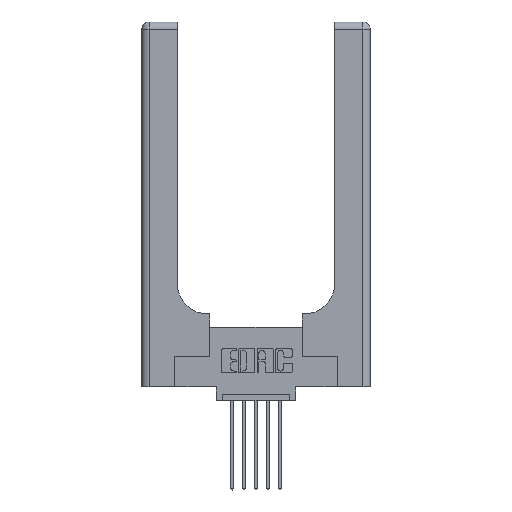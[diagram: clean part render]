
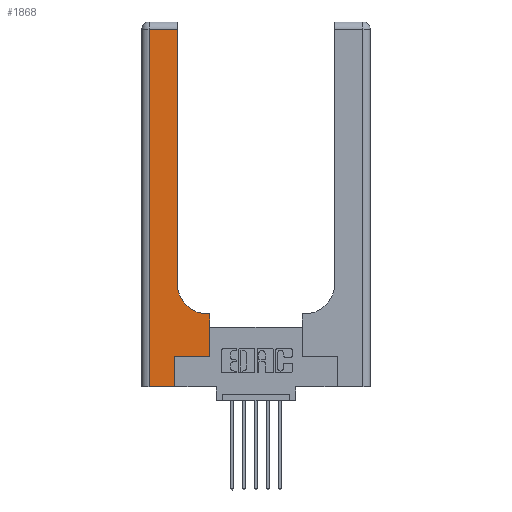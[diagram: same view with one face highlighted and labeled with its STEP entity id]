
A CAD part, top view. The second image highlights one B-rep face of the part: STEP entity #1868.
In plain terms, the highlighted planar face has unit normal (0, 0, 1).
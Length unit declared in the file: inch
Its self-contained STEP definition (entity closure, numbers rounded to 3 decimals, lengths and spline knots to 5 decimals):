
#275 = VERTEX_POINT ( 'NONE', #4577 ) ;
#542 = VECTOR ( 'NONE', #3046, 39.37008 ) ;
#587 = VERTEX_POINT ( 'NONE', #5018 ) ;
#690 = CARTESIAN_POINT ( 'NONE',  ( 0.269, 0.25, 0.37 ) ) ;
#755 = CARTESIAN_POINT ( 'NONE',  ( 0.2915, 0.6, 0.37 ) ) ;
#831 = CARTESIAN_POINT ( 'NONE',  ( 0.269, 0., 0.37 ) ) ;
#941 = CARTESIAN_POINT ( 'NONE',  ( 0.2915, 3., 0.37 ) ) ;
#1002 = DIRECTION ( 'NONE',  ( 0., 0., -1. ) ) ;
#1436 = DIRECTION ( 'NONE',  ( -1., 0., 0. ) ) ;
#1779 = LINE ( 'NONE', #690, #10095 ) ;
#1868 = ADVANCED_FACE ( 'NONE', ( #9483 ), #13088, .F. ) ;
#1995 = CARTESIAN_POINT ( 'NONE',  ( 0., 0., 0.37 ) ) ;
#2372 = CARTESIAN_POINT ( 'NONE',  ( 0.5585, 0.25, 0.37 ) ) ;
#2535 = LINE ( 'NONE', #12269, #5595 ) ;
#2660 = VECTOR ( 'NONE', #11722, 39.37008 ) ;
#2912 = CARTESIAN_POINT ( 'NONE',  ( 0.06, 3., 0.37 ) ) ;
#2940 = ORIENTED_EDGE ( 'NONE', *, *, #10793, .T. ) ;
#3046 = DIRECTION ( 'NONE',  ( 0., -1., 0. ) ) ;
#3082 = EDGE_CURVE ( 'NONE', #13131, #10066, #3353, .T. ) ;
#3353 = LINE ( 'NONE', #941, #12027 ) ;
#3459 = LINE ( 'NONE', #2912, #542 ) ;
#3684 = ORIENTED_EDGE ( 'NONE', *, *, #12193, .T. ) ;
#4307 = DIRECTION ( 'NONE',  ( -1., 0., 0. ) ) ;
#4357 = CARTESIAN_POINT ( 'NONE',  ( 0., 3., 0.37 ) ) ;
#4577 = CARTESIAN_POINT ( 'NONE',  ( 0.06, 2.94, 0.37 ) ) ;
#4827 = EDGE_CURVE ( 'NONE', #5425, #5295, #1779, .T. ) ;
#5018 = CARTESIAN_POINT ( 'NONE',  ( 0.06, 0., 0.37 ) ) ;
#5270 = ORIENTED_EDGE ( 'NONE', *, *, #3082, .T. ) ;
#5295 = VERTEX_POINT ( 'NONE', #2372 ) ;
#5388 = ORIENTED_EDGE ( 'NONE', *, *, #13909, .T. ) ;
#5425 = VERTEX_POINT ( 'NONE', #6947 ) ;
#5511 = EDGE_CURVE ( 'NONE', #8713, #7028, #11079, .T. ) ;
#5540 = CARTESIAN_POINT ( 'NONE',  ( 0.269, 0., 0.37 ) ) ;
#5595 = VECTOR ( 'NONE', #1436, 39.37008 ) ;
#5997 = VECTOR ( 'NONE', #9329, 39.37008 ) ;
#6006 = ORIENTED_EDGE ( 'NONE', *, *, #4827, .T. ) ;
#6125 = ORIENTED_EDGE ( 'NONE', *, *, #5511, .T. ) ;
#6775 = ORIENTED_EDGE ( 'NONE', *, *, #10360, .T. ) ;
#6947 = CARTESIAN_POINT ( 'NONE',  ( 0.269, 0.25, 0.37 ) ) ;
#7028 = VERTEX_POINT ( 'NONE', #7727 ) ;
#7497 = EDGE_CURVE ( 'NONE', #7028, #13131, #9045, .T. ) ;
#7557 = LINE ( 'NONE', #5540, #11833 ) ;
#7727 = CARTESIAN_POINT ( 'NONE',  ( 0.5415, 0.6, 0.37 ) ) ;
#8270 = LINE ( 'NONE', #1995, #2660 ) ;
#8499 = AXIS2_PLACEMENT_3D ( 'NONE', #4357, #1002, #4307 ) ;
#8713 = VERTEX_POINT ( 'NONE', #13704 ) ;
#8810 = ORIENTED_EDGE ( 'NONE', *, *, #7497, .T. ) ;
#9045 = CIRCLE ( 'NONE', #9625, 0.25 ) ;
#9074 = CARTESIAN_POINT ( 'NONE',  ( 0.5585, 0.25, 0.37 ) ) ;
#9208 = DIRECTION ( 'NONE',  ( 0., 0., -1. ) ) ;
#9329 = DIRECTION ( 'NONE',  ( -1., 0., 0. ) ) ;
#9414 = EDGE_LOOP ( 'NONE', ( #5270, #2940, #5388, #3684, #9775, #6006, #6775, #6125, #8810 ) ) ;
#9472 = DIRECTION ( 'NONE',  ( 0., 1., 0. ) ) ;
#9483 = FACE_OUTER_BOUND ( 'NONE', #9414, .T. ) ;
#9625 = AXIS2_PLACEMENT_3D ( 'NONE', #10216, #9208, #13490 ) ;
#9775 = ORIENTED_EDGE ( 'NONE', *, *, #12348, .T. ) ;
#10066 = VERTEX_POINT ( 'NONE', #13756 ) ;
#10095 = VECTOR ( 'NONE', #13627, 39.37008 ) ;
#10216 = CARTESIAN_POINT ( 'NONE',  ( 0.5415, 0.85, 0.37 ) ) ;
#10360 = EDGE_CURVE ( 'NONE', #5295, #8713, #12574, .T. ) ;
#10793 = EDGE_CURVE ( 'NONE', #10066, #275, #2535, .T. ) ;
#11029 = VECTOR ( 'NONE', #12369, 39.37008 ) ;
#11079 = LINE ( 'NONE', #755, #5997 ) ;
#11722 = DIRECTION ( 'NONE',  ( 1., 0., 0. ) ) ;
#11833 = VECTOR ( 'NONE', #13087, 39.37008 ) ;
#12027 = VECTOR ( 'NONE', #9472, 39.37008 ) ;
#12193 = EDGE_CURVE ( 'NONE', #587, #13829, #8270, .T. ) ;
#12256 = CARTESIAN_POINT ( 'NONE',  ( 0.2915, 0.85, 0.37 ) ) ;
#12269 = CARTESIAN_POINT ( 'NONE',  ( 0., 2.94, 0.37 ) ) ;
#12348 = EDGE_CURVE ( 'NONE', #13829, #5425, #7557, .T. ) ;
#12369 = DIRECTION ( 'NONE',  ( 0., 1., 0. ) ) ;
#12574 = LINE ( 'NONE', #9074, #11029 ) ;
#13087 = DIRECTION ( 'NONE',  ( 0., 1., 0. ) ) ;
#13088 = PLANE ( 'NONE',  #8499 ) ;
#13131 = VERTEX_POINT ( 'NONE', #12256 ) ;
#13490 = DIRECTION ( 'NONE',  ( 1., 0., 0. ) ) ;
#13627 = DIRECTION ( 'NONE',  ( 1., 0., 0. ) ) ;
#13704 = CARTESIAN_POINT ( 'NONE',  ( 0.5585, 0.6, 0.37 ) ) ;
#13756 = CARTESIAN_POINT ( 'NONE',  ( 0.2915, 2.94, 0.37 ) ) ;
#13829 = VERTEX_POINT ( 'NONE', #831 ) ;
#13909 = EDGE_CURVE ( 'NONE', #275, #587, #3459, .T. ) ;
